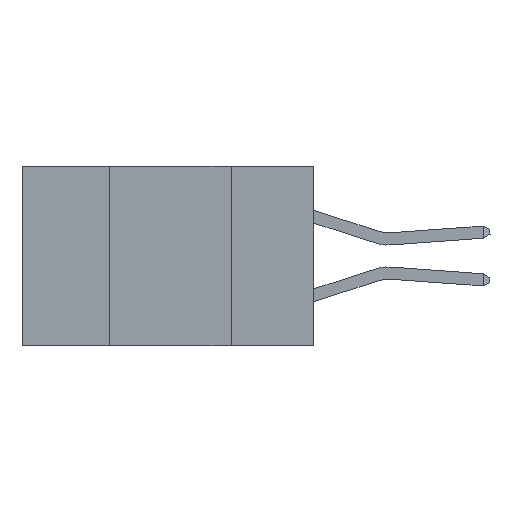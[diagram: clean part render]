
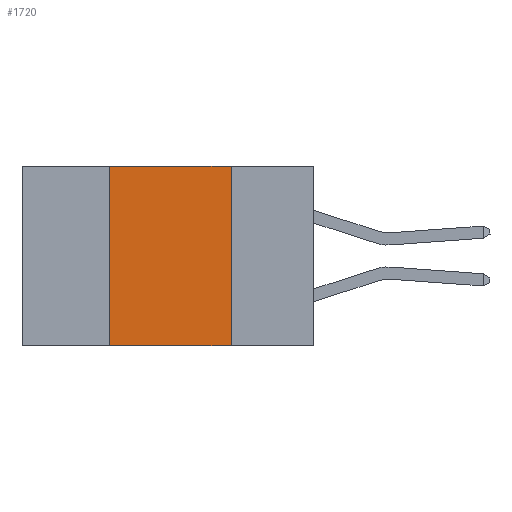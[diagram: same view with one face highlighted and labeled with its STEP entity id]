
A CAD part, left-side view. The second image highlights one B-rep face of the part: STEP entity #1720.
In plain terms, the highlighted planar face has unit normal (-1, 0, 0).
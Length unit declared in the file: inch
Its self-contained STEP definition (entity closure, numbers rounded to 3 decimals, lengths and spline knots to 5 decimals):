
#725 = VERTEX_POINT ( 'NONE', #6157 ) ;
#1267 = AXIS2_PLACEMENT_3D ( 'NONE', #18367, #20564, #7362 ) ;
#1527 = FACE_OUTER_BOUND ( 'NONE', #6304, .T. ) ;
#1720 = ADVANCED_FACE ( 'NONE', ( #1527 ), #5119, .F. ) ;
#1957 = EDGE_CURVE ( 'NONE', #9966, #2094, #18113, .T. ) ;
#2094 = VERTEX_POINT ( 'NONE', #23807 ) ;
#2500 = ORIENTED_EDGE ( 'NONE', *, *, #15914, .F. ) ;
#2608 = CARTESIAN_POINT ( 'NONE',  ( 0., 0.6, -0.37 ) ) ;
#3895 = ORIENTED_EDGE ( 'NONE', *, *, #1957, .F. ) ;
#4577 = ORIENTED_EDGE ( 'NONE', *, *, #20251, .T. ) ;
#5119 = PLANE ( 'NONE',  #1267 ) ;
#5134 = CARTESIAN_POINT ( 'NONE',  ( 0., 0.6, 0. ) ) ;
#5540 = CARTESIAN_POINT ( 'NONE',  ( 0., 0.42, -0.37 ) ) ;
#6157 = CARTESIAN_POINT ( 'NONE',  ( 0., 0.17, -0.37 ) ) ;
#6304 = EDGE_LOOP ( 'NONE', ( #23875, #2500, #3895, #4577 ) ) ;
#6375 = VECTOR ( 'NONE', #25594, 39.37008 ) ;
#6408 = EDGE_CURVE ( 'NONE', #27335, #725, #28286, .T. ) ;
#7362 = DIRECTION ( 'NONE',  ( 0., 0., -1. ) ) ;
#8037 = CARTESIAN_POINT ( 'NONE',  ( 0., 0.42, 0. ) ) ;
#9966 = VERTEX_POINT ( 'NONE', #5540 ) ;
#11471 = LINE ( 'NONE', #2608, #28241 ) ;
#12205 = VECTOR ( 'NONE', #12859, 39.37008 ) ;
#12859 = DIRECTION ( 'NONE',  ( 0., 0., -1. ) ) ;
#15914 = EDGE_CURVE ( 'NONE', #2094, #27335, #20663, .T. ) ;
#16170 = DIRECTION ( 'NONE',  ( 0., -1., 0. ) ) ;
#18061 = DIRECTION ( 'NONE',  ( 0., -1., 0. ) ) ;
#18113 = LINE ( 'NONE', #8037, #6375 ) ;
#18367 = CARTESIAN_POINT ( 'NONE',  ( 0., 0.6, 0. ) ) ;
#20251 = EDGE_CURVE ( 'NONE', #9966, #725, #11471, .T. ) ;
#20564 = DIRECTION ( 'NONE',  ( 1., 0., 0. ) ) ;
#20663 = LINE ( 'NONE', #5134, #25780 ) ;
#23807 = CARTESIAN_POINT ( 'NONE',  ( 0., 0.42, 0. ) ) ;
#23875 = ORIENTED_EDGE ( 'NONE', *, *, #6408, .F. ) ;
#25594 = DIRECTION ( 'NONE',  ( 0., 0., 1. ) ) ;
#25780 = VECTOR ( 'NONE', #16170, 39.37008 ) ;
#26394 = CARTESIAN_POINT ( 'NONE',  ( 0., 0.17, 0. ) ) ;
#27335 = VERTEX_POINT ( 'NONE', #27554 ) ;
#27554 = CARTESIAN_POINT ( 'NONE',  ( 0., 0.17, 0. ) ) ;
#28241 = VECTOR ( 'NONE', #18061, 39.37008 ) ;
#28286 = LINE ( 'NONE', #26394, #12205 ) ;
